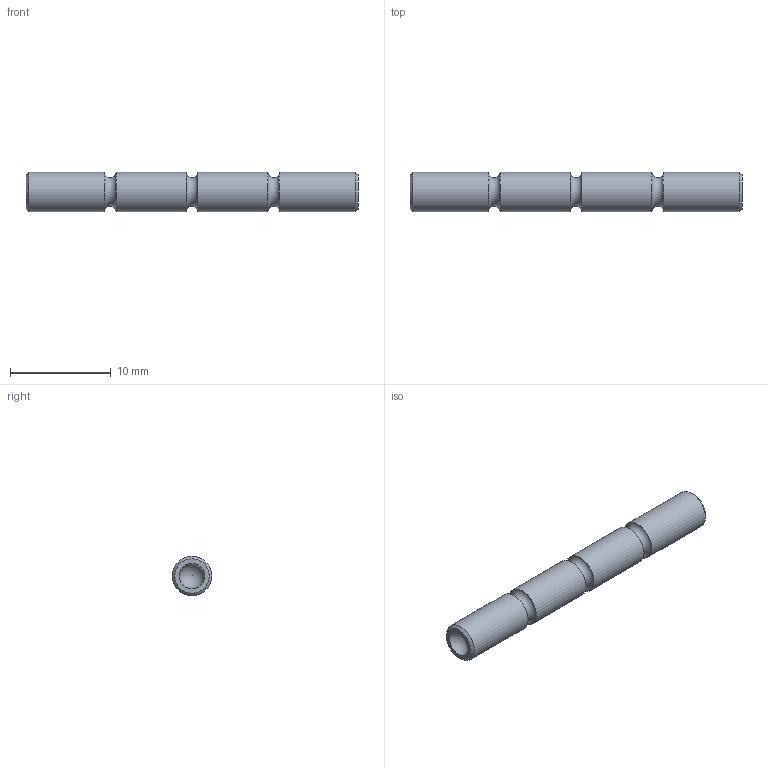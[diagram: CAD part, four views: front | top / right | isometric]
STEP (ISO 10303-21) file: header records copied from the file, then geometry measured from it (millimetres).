
FILE_DESCRIPTION(/* description */ (''),/* implementation_level */ '2;1');
FILE_NAME(/* name */ 'Rem Pin v2.step',/* time_stamp */ '2021-04-20T06:57:32-05:00',/* author */ (''),/* organization */ (''),/* preprocessor_version */ 'ST-DEVELOPER v18.1',/* originating_system */ 'Autodesk Translation Framework v10.6.0.1341',/* authorisation */ '');
FILE_SCHEMA (('AUTOMOTIVE_DESIGN { 1 0 10303 214 3 1 1 }'));
Length unit declared in the file: inch
Products named in the file (1): Rem Pin
Bounding box: 33.02 x 3.92 x 3.92 mm (x, y, z)
Volume: 374 mm3; surface area: 448.6 mm2
Topology: 1 solids, 1 shells, 13 faces, 27 edges, 16 vertices
Faces by surface type: cylinder 4, torus 3, cone 2, plane 2, sphere 2
Full cylindrical faces by diameter (mm): 3.924 x4
Entity records: 377 total; most frequent: DIRECTION 72, CARTESIAN_POINT 55, ORIENTED_EDGE 50, AXIS2_PLACEMENT_3D 33, EDGE_CURVE 25, CIRCLE 19, VERTEX_POINT 16, EDGE_LOOP 15
